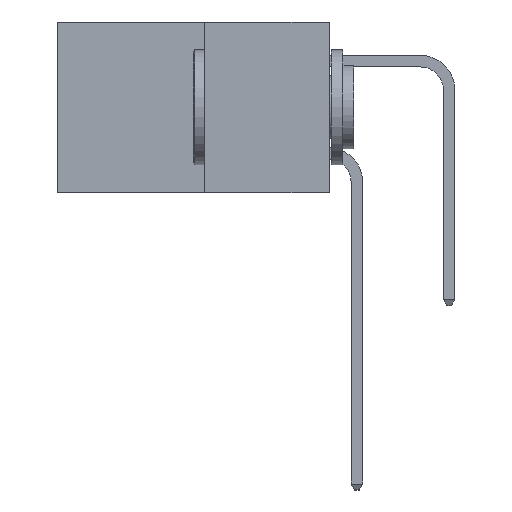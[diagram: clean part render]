
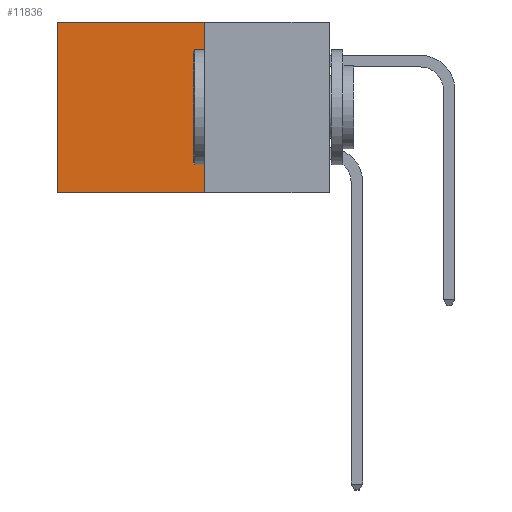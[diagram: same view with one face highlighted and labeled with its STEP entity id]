
A CAD part, left-side view. The second image highlights one B-rep face of the part: STEP entity #11836.
In plain terms, the highlighted planar face has unit normal (-1, 0, 0).
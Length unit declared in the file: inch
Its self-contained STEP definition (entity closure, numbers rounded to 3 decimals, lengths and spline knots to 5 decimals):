
#208 = ORIENTED_EDGE ( 'NONE', *, *, #8535, .F. ) ;
#1018 = CARTESIAN_POINT ( 'NONE',  ( 0.277, 0.59, 0. ) ) ;
#1230 = VECTOR ( 'NONE', #6219, 39.37008 ) ;
#2154 = EDGE_CURVE ( 'NONE', #2787, #12405, #6710, .T. ) ;
#2192 = CARTESIAN_POINT ( 'NONE',  ( 0.277, 0.27, -0.37 ) ) ;
#2378 = CARTESIAN_POINT ( 'NONE',  ( 0.277, 0.27, -0.37 ) ) ;
#2787 = VERTEX_POINT ( 'NONE', #11627 ) ;
#2838 = CARTESIAN_POINT ( 'NONE',  ( 0.277, 0.59, -0.37 ) ) ;
#2844 = AXIS2_PLACEMENT_3D ( 'NONE', #2378, #10691, #4419 ) ;
#2907 = VERTEX_POINT ( 'NONE', #10903 ) ;
#3104 = CARTESIAN_POINT ( 'NONE',  ( 0.277, 0.27, -0.37 ) ) ;
#3188 = ORIENTED_EDGE ( 'NONE', *, *, #5959, .T. ) ;
#3397 = PLANE ( 'NONE',  #2844 ) ;
#3824 = DIRECTION ( 'NONE',  ( 0., 0., -1. ) ) ;
#3884 = VECTOR ( 'NONE', #12293, 39.37008 ) ;
#3959 = LINE ( 'NONE', #9469, #1230 ) ;
#4419 = DIRECTION ( 'NONE',  ( 0., 0., -1. ) ) ;
#4560 = VECTOR ( 'NONE', #12502, 39.37008 ) ;
#5341 = EDGE_CURVE ( 'NONE', #2787, #6997, #7447, .T. ) ;
#5904 = CARTESIAN_POINT ( 'NONE',  ( 0.277, 0.27, 0. ) ) ;
#5959 = EDGE_CURVE ( 'NONE', #6997, #2907, #7767, .T. ) ;
#6219 = DIRECTION ( 'NONE',  ( 0., 1., 0. ) ) ;
#6430 = ORIENTED_EDGE ( 'NONE', *, *, #2154, .F. ) ;
#6710 = LINE ( 'NONE', #2192, #3884 ) ;
#6997 = VERTEX_POINT ( 'NONE', #1018 ) ;
#7447 = LINE ( 'NONE', #5904, #4560 ) ;
#7767 = LINE ( 'NONE', #2838, #12440 ) ;
#7814 = EDGE_LOOP ( 'NONE', ( #3188, #208, #6430, #7892 ) ) ;
#7892 = ORIENTED_EDGE ( 'NONE', *, *, #5341, .T. ) ;
#8535 = EDGE_CURVE ( 'NONE', #12405, #2907, #3959, .T. ) ;
#9469 = CARTESIAN_POINT ( 'NONE',  ( 0.277, 0.27, -0.37 ) ) ;
#10691 = DIRECTION ( 'NONE',  ( 1., 0., 0. ) ) ;
#10903 = CARTESIAN_POINT ( 'NONE',  ( 0.277, 0.59, -0.37 ) ) ;
#11627 = CARTESIAN_POINT ( 'NONE',  ( 0.277, 0.27, 0. ) ) ;
#11836 = ADVANCED_FACE ( 'NONE', ( #12467 ), #3397, .F. ) ;
#12293 = DIRECTION ( 'NONE',  ( 0., 0., -1. ) ) ;
#12405 = VERTEX_POINT ( 'NONE', #3104 ) ;
#12440 = VECTOR ( 'NONE', #3824, 39.37008 ) ;
#12467 = FACE_OUTER_BOUND ( 'NONE', #7814, .T. ) ;
#12502 = DIRECTION ( 'NONE',  ( 0., 1., 0. ) ) ;
